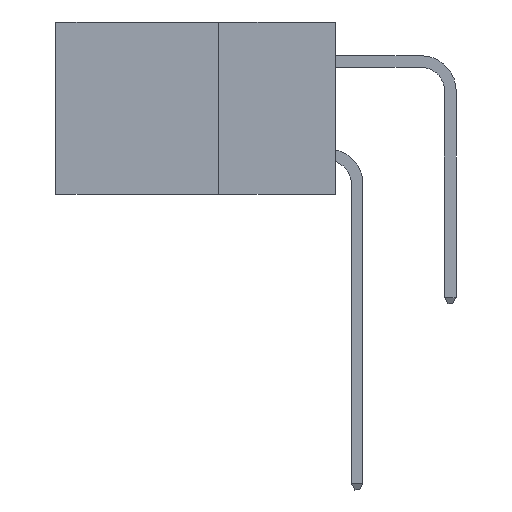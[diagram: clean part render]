
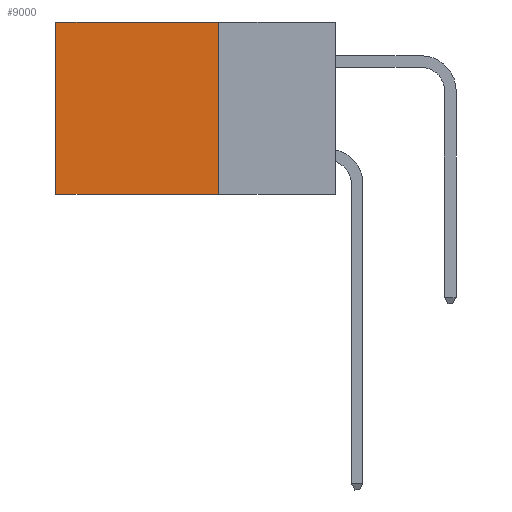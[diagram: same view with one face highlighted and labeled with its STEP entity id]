
A CAD part, left-side view. The second image highlights one B-rep face of the part: STEP entity #9000.
In plain terms, the highlighted planar face has unit normal (-1, 0, 0).
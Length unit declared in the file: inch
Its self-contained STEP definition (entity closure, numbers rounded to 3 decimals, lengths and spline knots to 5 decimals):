
#227 = VERTEX_POINT ( 'NONE', #24827 ) ;
#1087 = ORIENTED_EDGE ( 'NONE', *, *, #29200, .T. ) ;
#1442 = ORIENTED_EDGE ( 'NONE', *, *, #23104, .T. ) ;
#1807 = CARTESIAN_POINT ( 'NONE',  ( 0.2875, 0.25, 0. ) ) ;
#1986 = VECTOR ( 'NONE', #4227, 39.37008 ) ;
#2999 = DIRECTION ( 'NONE',  ( 0., 1., 0. ) ) ;
#3232 = CARTESIAN_POINT ( 'NONE',  ( 0.2875, 0.25, -0.37 ) ) ;
#4013 = VECTOR ( 'NONE', #2999, 39.37008 ) ;
#4227 = DIRECTION ( 'NONE',  ( 0., 0., -1. ) ) ;
#5694 = AXIS2_PLACEMENT_3D ( 'NONE', #22816, #29731, #10884 ) ;
#7210 = VERTEX_POINT ( 'NONE', #20252 ) ;
#8169 = EDGE_LOOP ( 'NONE', ( #1442, #15124, #29508, #1087 ) ) ;
#8226 = CARTESIAN_POINT ( 'NONE',  ( 0.2875, 0.6, 0. ) ) ;
#8441 = VECTOR ( 'NONE', #21666, 39.37008 ) ;
#8841 = LINE ( 'NONE', #3232, #4013 ) ;
#9000 = ADVANCED_FACE ( 'NONE', ( #28127 ), #27386, .F. ) ;
#10884 = DIRECTION ( 'NONE',  ( 0., 0., -1. ) ) ;
#10911 = DIRECTION ( 'NONE',  ( 0., 0., -1. ) ) ;
#14813 = CARTESIAN_POINT ( 'NONE',  ( 0.2875, 0.25, 0. ) ) ;
#15124 = ORIENTED_EDGE ( 'NONE', *, *, #20700, .F. ) ;
#15615 = EDGE_CURVE ( 'NONE', #20759, #227, #23167, .T. ) ;
#17421 = CARTESIAN_POINT ( 'NONE',  ( 0.2875, 0.25, 0. ) ) ;
#17577 = VECTOR ( 'NONE', #10911, 39.37008 ) ;
#20252 = CARTESIAN_POINT ( 'NONE',  ( 0.2875, 0.6, -0.37 ) ) ;
#20700 = EDGE_CURVE ( 'NONE', #227, #7210, #8841, .T. ) ;
#20759 = VERTEX_POINT ( 'NONE', #17421 ) ;
#21666 = DIRECTION ( 'NONE',  ( 0., 1., 0. ) ) ;
#22816 = CARTESIAN_POINT ( 'NONE',  ( 0.2875, 0.25, 0. ) ) ;
#23104 = EDGE_CURVE ( 'NONE', #27012, #7210, #29820, .T. ) ;
#23167 = LINE ( 'NONE', #1807, #1986 ) ;
#24827 = CARTESIAN_POINT ( 'NONE',  ( 0.2875, 0.25, -0.37 ) ) ;
#25507 = LINE ( 'NONE', #14813, #8441 ) ;
#27012 = VERTEX_POINT ( 'NONE', #28441 ) ;
#27386 = PLANE ( 'NONE',  #5694 ) ;
#28127 = FACE_OUTER_BOUND ( 'NONE', #8169, .T. ) ;
#28441 = CARTESIAN_POINT ( 'NONE',  ( 0.2875, 0.6, 0. ) ) ;
#29200 = EDGE_CURVE ( 'NONE', #20759, #27012, #25507, .T. ) ;
#29508 = ORIENTED_EDGE ( 'NONE', *, *, #15615, .F. ) ;
#29731 = DIRECTION ( 'NONE',  ( 1., 0., 0. ) ) ;
#29820 = LINE ( 'NONE', #8226, #17577 ) ;
